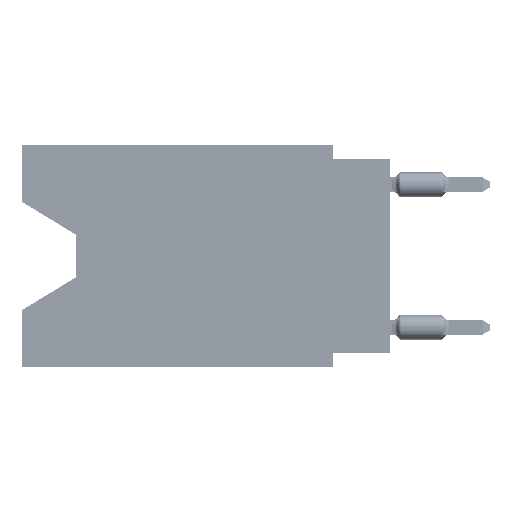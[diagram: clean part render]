
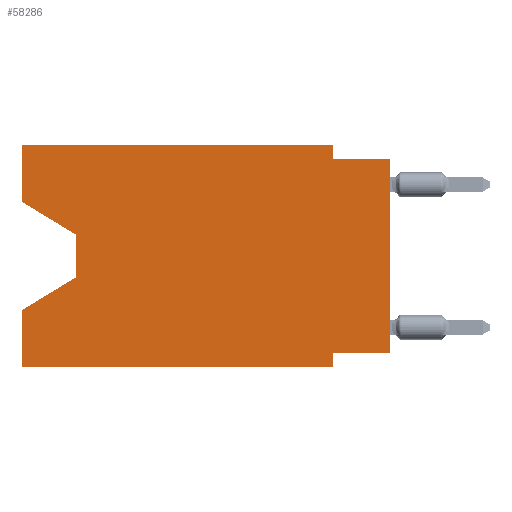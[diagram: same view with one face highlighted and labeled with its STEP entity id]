
A CAD part, left-side view. The second image highlights one B-rep face of the part: STEP entity #58286.
In plain terms, the highlighted planar face has unit normal (-1, 0, 0).
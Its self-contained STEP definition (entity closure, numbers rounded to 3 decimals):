
#916 = EDGE_CURVE ( 'NONE', #7495, #40422, #32142, .T. ) ;
#1785 = DIRECTION ( 'NONE',  ( 0., -0.855, -0.519 ) ) ;
#2762 = LINE ( 'NONE', #34783, #41700 ) ;
#2838 = VECTOR ( 'NONE', #55344, 1000. ) ;
#2922 = CARTESIAN_POINT ( 'NONE',  ( 0., 13.97, -5.893 ) ) ;
#3208 = VERTEX_POINT ( 'NONE', #14276 ) ;
#3605 = VERTEX_POINT ( 'NONE', #53407 ) ;
#3693 = ORIENTED_EDGE ( 'NONE', *, *, #5569, .F. ) ;
#4372 = VERTEX_POINT ( 'NONE', #28792 ) ;
#5466 = VECTOR ( 'NONE', #7589, 1000. ) ;
#5569 = EDGE_CURVE ( 'NONE', #40422, #24957, #35455, .T. ) ;
#6470 = ORIENTED_EDGE ( 'NONE', *, *, #26017, .T. ) ;
#6488 = CARTESIAN_POINT ( 'NONE',  ( 0., 2.54, -9.271 ) ) ;
#7495 = VERTEX_POINT ( 'NONE', #37954 ) ;
#7589 = DIRECTION ( 'NONE',  ( 0., 0., 1. ) ) ;
#8230 = VERTEX_POINT ( 'NONE', #55104 ) ;
#8254 = ORIENTED_EDGE ( 'NONE', *, *, #9751, .F. ) ;
#8968 = CARTESIAN_POINT ( 'NONE',  ( 0., 16.383, 0. ) ) ;
#9321 = LINE ( 'NONE', #60476, #14947 ) ;
#9420 = VECTOR ( 'NONE', #66557, 1000. ) ;
#9751 = EDGE_CURVE ( 'NONE', #8230, #7495, #2762, .T. ) ;
#10522 = VERTEX_POINT ( 'NONE', #63399 ) ;
#11491 = ORIENTED_EDGE ( 'NONE', *, *, #37484, .T. ) ;
#12737 = VERTEX_POINT ( 'NONE', #6488 ) ;
#14269 = DIRECTION ( 'NONE',  ( 0., 0., 1. ) ) ;
#14276 = CARTESIAN_POINT ( 'NONE',  ( 0., 16.383, -7.36 ) ) ;
#14947 = VECTOR ( 'NONE', #49015, 1000. ) ;
#15364 = CARTESIAN_POINT ( 'NONE',  ( 0., 2.54, 0. ) ) ;
#17764 = EDGE_CURVE ( 'NONE', #3605, #12737, #72841, .T. ) ;
#21435 = VERTEX_POINT ( 'NONE', #2922 ) ;
#21753 = CARTESIAN_POINT ( 'NONE',  ( 0., 0., -9.271 ) ) ;
#22004 = LINE ( 'NONE', #44605, #2838 ) ;
#22094 = DIRECTION ( 'NONE',  ( 0., 0.855, -0.519 ) ) ;
#23817 = ORIENTED_EDGE ( 'NONE', *, *, #54539, .F. ) ;
#24185 = EDGE_CURVE ( 'NONE', #44560, #3208, #42701, .T. ) ;
#24957 = VERTEX_POINT ( 'NONE', #63644 ) ;
#25123 = DIRECTION ( 'NONE',  ( 0., 0., 1. ) ) ;
#25835 = EDGE_CURVE ( 'NONE', #26585, #21435, #9321, .T. ) ;
#26017 = EDGE_CURVE ( 'NONE', #3605, #4372, #35882, .T. ) ;
#26585 = VERTEX_POINT ( 'NONE', #66142 ) ;
#27771 = CARTESIAN_POINT ( 'NONE',  ( 0., 0., -0.635 ) ) ;
#27916 = ORIENTED_EDGE ( 'NONE', *, *, #43118, .T. ) ;
#28792 = CARTESIAN_POINT ( 'NONE',  ( 0., 0., -0.635 ) ) ;
#30496 = FACE_OUTER_BOUND ( 'NONE', #72935, .T. ) ;
#32135 = ORIENTED_EDGE ( 'NONE', *, *, #47243, .T. ) ;
#32142 = LINE ( 'NONE', #50318, #49236 ) ;
#33618 = DIRECTION ( 'NONE',  ( 0., -1., 0. ) ) ;
#34723 = CARTESIAN_POINT ( 'NONE',  ( 0., 2.54, 0. ) ) ;
#34783 = CARTESIAN_POINT ( 'NONE',  ( 0., 16.383, 0. ) ) ;
#35455 = LINE ( 'NONE', #34723, #40222 ) ;
#35882 = LINE ( 'NONE', #37335, #72902 ) ;
#36780 = ORIENTED_EDGE ( 'NONE', *, *, #45814, .F. ) ;
#37335 = CARTESIAN_POINT ( 'NONE',  ( 0., 0., 0. ) ) ;
#37484 = EDGE_CURVE ( 'NONE', #21435, #3208, #45071, .T. ) ;
#37954 = CARTESIAN_POINT ( 'NONE',  ( 0., 16.383, 0. ) ) ;
#40222 = VECTOR ( 'NONE', #52529, 1000. ) ;
#40422 = VERTEX_POINT ( 'NONE', #15364 ) ;
#40600 = CARTESIAN_POINT ( 'NONE',  ( 0., 16.383, 0. ) ) ;
#40878 = ORIENTED_EDGE ( 'NONE', *, *, #916, .F. ) ;
#41102 = CARTESIAN_POINT ( 'NONE',  ( 0., 16.383, -2.546 ) ) ;
#41700 = VECTOR ( 'NONE', #14269, 1000. ) ;
#42701 = LINE ( 'NONE', #40600, #5466 ) ;
#43118 = EDGE_CURVE ( 'NONE', #8230, #26585, #69233, .T. ) ;
#44560 = VERTEX_POINT ( 'NONE', #49594 ) ;
#44605 = CARTESIAN_POINT ( 'NONE',  ( 0., 16.383, -9.906 ) ) ;
#45071 = LINE ( 'NONE', #67638, #45542 ) ;
#45542 = VECTOR ( 'NONE', #22094, 1000. ) ;
#45814 = EDGE_CURVE ( 'NONE', #12737, #10522, #61528, .T. ) ;
#47243 = EDGE_CURVE ( 'NONE', #44560, #10522, #22004, .T. ) ;
#49015 = DIRECTION ( 'NONE',  ( 0., 0., -1. ) ) ;
#49236 = VECTOR ( 'NONE', #33618, 1000. ) ;
#49594 = CARTESIAN_POINT ( 'NONE',  ( 0., 16.383, -9.906 ) ) ;
#50318 = CARTESIAN_POINT ( 'NONE',  ( 0., 16.383, 0. ) ) ;
#52099 = VECTOR ( 'NONE', #68130, 1000. ) ;
#52529 = DIRECTION ( 'NONE',  ( 0., 0., -1. ) ) ;
#53407 = CARTESIAN_POINT ( 'NONE',  ( 0., 0., -9.271 ) ) ;
#54539 = EDGE_CURVE ( 'NONE', #24957, #4372, #54947, .T. ) ;
#54947 = LINE ( 'NONE', #27771, #52099 ) ;
#55104 = CARTESIAN_POINT ( 'NONE',  ( 0., 16.383, -2.546 ) ) ;
#55344 = DIRECTION ( 'NONE',  ( 0., -1., 0. ) ) ;
#55349 = ORIENTED_EDGE ( 'NONE', *, *, #17764, .F. ) ;
#56773 = ORIENTED_EDGE ( 'NONE', *, *, #24185, .F. ) ;
#58286 = ADVANCED_FACE ( 'NONE', ( #30496 ), #70472, .F. ) ;
#60057 = DIRECTION ( 'NONE',  ( 0., 0., -1. ) ) ;
#60476 = CARTESIAN_POINT ( 'NONE',  ( 0., 13.97, -4.013 ) ) ;
#60798 = CARTESIAN_POINT ( 'NONE',  ( 0., 2.54, -9.906 ) ) ;
#61363 = AXIS2_PLACEMENT_3D ( 'NONE', #8968, #70113, #65659 ) ;
#61528 = LINE ( 'NONE', #60798, #65592 ) ;
#61799 = VECTOR ( 'NONE', #1785, 1000. ) ;
#63399 = CARTESIAN_POINT ( 'NONE',  ( 0., 2.54, -9.906 ) ) ;
#63644 = CARTESIAN_POINT ( 'NONE',  ( 0., 2.54, -0.635 ) ) ;
#65592 = VECTOR ( 'NONE', #60057, 1000. ) ;
#65659 = DIRECTION ( 'NONE',  ( 0., 0., -1. ) ) ;
#66142 = CARTESIAN_POINT ( 'NONE',  ( 0., 13.97, -4.013 ) ) ;
#66557 = DIRECTION ( 'NONE',  ( 0., 1., 0. ) ) ;
#67638 = CARTESIAN_POINT ( 'NONE',  ( 0., 13.97, -5.893 ) ) ;
#68130 = DIRECTION ( 'NONE',  ( 0., -1., 0. ) ) ;
#69233 = LINE ( 'NONE', #41102, #61799 ) ;
#70113 = DIRECTION ( 'NONE',  ( 1., 0., 0. ) ) ;
#70472 = PLANE ( 'NONE',  #61363 ) ;
#72167 = ORIENTED_EDGE ( 'NONE', *, *, #25835, .T. ) ;
#72841 = LINE ( 'NONE', #21753, #9420 ) ;
#72902 = VECTOR ( 'NONE', #25123, 1000. ) ;
#72935 = EDGE_LOOP ( 'NONE', ( #27916, #72167, #11491, #56773, #32135, #36780, #55349, #6470, #23817, #3693, #40878, #8254 ) ) ;
